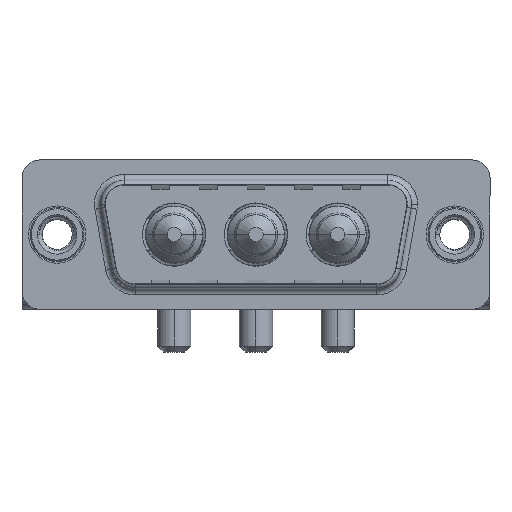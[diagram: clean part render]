
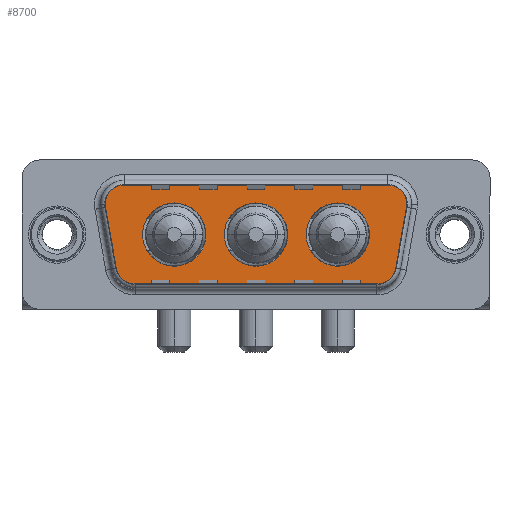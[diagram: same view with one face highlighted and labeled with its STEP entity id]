
A CAD part, top view. The second image highlights one B-rep face of the part: STEP entity #8700.
In plain terms, the highlighted planar face has unit normal (0, 0, 1).
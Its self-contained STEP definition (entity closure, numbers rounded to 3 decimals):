
#9 = CARTESIAN_POINT ( 'NONE',  ( 23.5, 0., 0. ) ) ;
#23 = CARTESIAN_POINT ( 'NONE',  ( 29.859, 2.553, 0. ) ) ;
#68 = CARTESIAN_POINT ( 'NONE',  ( 7.15, 0., 0. ) ) ;
#127 = CARTESIAN_POINT ( 'NONE',  ( 26.15, 0., 0. ) ) ;
#294 = DIRECTION ( 'NONE',  ( 0., 0., 1. ) ) ;
#381 = DIRECTION ( 'NONE',  ( 1., 0., 0. ) ) ;
#817 = EDGE_CURVE ( 'NONE', #10011, #8475, #13038, .T. ) ;
#833 = DIRECTION ( 'NONE',  ( 1., 0., 0. ) ) ;
#836 = EDGE_CURVE ( 'NONE', #10369, #5681, #14998, .T. ) ;
#904 = CIRCLE ( 'NONE', #12830, 2.65 ) ;
#1155 = AXIS2_PLACEMENT_3D ( 'NONE', #2225, #6966, #15307 ) ;
#1267 = CARTESIAN_POINT ( 'NONE',  ( 29.889, 2.9, 0. ) ) ;
#1299 = ORIENTED_EDGE ( 'NONE', *, *, #836, .T. ) ;
#1435 = CARTESIAN_POINT ( 'NONE',  ( 26.866, -4.9, 0. ) ) ;
#1461 = ORIENTED_EDGE ( 'NONE', *, *, #11948, .T. ) ;
#1512 = CIRCLE ( 'NONE', #6464, 2. ) ;
#1799 = EDGE_LOOP ( 'NONE', ( #3081, #1461, #11529, #5918, #14019, #12691, #6817, #14729, #1299 ) ) ;
#1834 = VERTEX_POINT ( 'NONE', #5460 ) ;
#1970 = EDGE_CURVE ( 'NONE', #3866, #10369, #1512, .T. ) ;
#2027 = VERTEX_POINT ( 'NONE', #13457 ) ;
#2169 = CARTESIAN_POINT ( 'NONE',  ( 5.411, 4.9, 0. ) ) ;
#2188 = AXIS2_PLACEMENT_3D ( 'NONE', #6352, #7614, #15015 ) ;
#2225 = CARTESIAN_POINT ( 'NONE',  ( 26.866, -2.9, 0. ) ) ;
#2233 = EDGE_CURVE ( 'NONE', #1834, #3443, #10955, .T. ) ;
#2374 = VECTOR ( 'NONE', #9341, 1000. ) ;
#2638 = CARTESIAN_POINT ( 'NONE',  ( 26.866, -2.9, 0. ) ) ;
#2776 = DIRECTION ( 'NONE',  ( 1., 0., 0. ) ) ;
#2869 = CARTESIAN_POINT ( 'NONE',  ( 19.3, 0., 0. ) ) ;
#3081 = ORIENTED_EDGE ( 'NONE', *, *, #5505, .T. ) ;
#3117 = ORIENTED_EDGE ( 'NONE', *, *, #9823, .F. ) ;
#3417 = DIRECTION ( 'NONE',  ( 0., 0., 1. ) ) ;
#3424 = CARTESIAN_POINT ( 'NONE',  ( 14., 0., 0. ) ) ;
#3443 = VERTEX_POINT ( 'NONE', #68 ) ;
#3513 = VERTEX_POINT ( 'NONE', #12124 ) ;
#3814 = FACE_BOUND ( 'NONE', #7966, .T. ) ;
#3866 = VERTEX_POINT ( 'NONE', #4338 ) ;
#3917 = CARTESIAN_POINT ( 'NONE',  ( 3.441, 2.553, 0. ) ) ;
#4032 = CARTESIAN_POINT ( 'NONE',  ( 5.411, 2.9, 0. ) ) ;
#4164 = VERTEX_POINT ( 'NONE', #4948 ) ;
#4166 = CIRCLE ( 'NONE', #2188, 2. ) ;
#4332 = CARTESIAN_POINT ( 'NONE',  ( 6.434, -4.9, 0. ) ) ;
#4338 = CARTESIAN_POINT ( 'NONE',  ( 4.464, -3.247, 0. ) ) ;
#4465 = CARTESIAN_POINT ( 'NONE',  ( 16.65, 0., 0. ) ) ;
#4595 = CARTESIAN_POINT ( 'NONE',  ( 6.434, -4.9, 0. ) ) ;
#4602 = CARTESIAN_POINT ( 'NONE',  ( 6.434, -2.9, 0. ) ) ;
#4746 = CARTESIAN_POINT ( 'NONE',  ( 16.65, 0., 0. ) ) ;
#4827 = CARTESIAN_POINT ( 'NONE',  ( 27.889, 4.9, 0. ) ) ;
#4946 = DIRECTION ( 'NONE',  ( 0.174, -0.985, 0. ) ) ;
#4948 = CARTESIAN_POINT ( 'NONE',  ( 20.85, 0., 0. ) ) ;
#4985 = EDGE_CURVE ( 'NONE', #13794, #3513, #14086, .T. ) ;
#5131 = CIRCLE ( 'NONE', #13845, 2.65 ) ;
#5460 = CARTESIAN_POINT ( 'NONE',  ( 12.45, 0., 0. ) ) ;
#5505 = EDGE_CURVE ( 'NONE', #5681, #9298, #15074, .T. ) ;
#5681 = VERTEX_POINT ( 'NONE', #1435 ) ;
#5796 = CARTESIAN_POINT ( 'NONE',  ( 27.889, 2.9, 0. ) ) ;
#5821 = DIRECTION ( 'NONE',  ( 1., 0., 0. ) ) ;
#5832 = AXIS2_PLACEMENT_3D ( 'NONE', #5796, #13989, #10556 ) ;
#5918 = ORIENTED_EDGE ( 'NONE', *, *, #12123, .T. ) ;
#5924 = DIRECTION ( 'NONE',  ( 0., 0., 1. ) ) ;
#5978 = AXIS2_PLACEMENT_3D ( 'NONE', #6756, #11443, #11521 ) ;
#6019 = EDGE_CURVE ( 'NONE', #3513, #2027, #15088, .T. ) ;
#6352 = CARTESIAN_POINT ( 'NONE',  ( 27.889, 2.9, 0. ) ) ;
#6464 = AXIS2_PLACEMENT_3D ( 'NONE', #4602, #5924, #9364 ) ;
#6468 = EDGE_CURVE ( 'NONE', #8916, #11478, #13773, .T. ) ;
#6756 = CARTESIAN_POINT ( 'NONE',  ( 9.8, 0., 0. ) ) ;
#6817 = ORIENTED_EDGE ( 'NONE', *, *, #7096, .T. ) ;
#6966 = DIRECTION ( 'NONE',  ( 0., 0., 1. ) ) ;
#7051 = AXIS2_PLACEMENT_3D ( 'NONE', #4746, #3417, #5821 ) ;
#7096 = EDGE_CURVE ( 'NONE', #2027, #3866, #8674, .T. ) ;
#7401 = DIRECTION ( 'NONE',  ( 0., 0., 1. ) ) ;
#7614 = DIRECTION ( 'NONE',  ( 0., 0., 1. ) ) ;
#7818 = CARTESIAN_POINT ( 'NONE',  ( 28.836, -3.247, 0. ) ) ;
#7966 = EDGE_LOOP ( 'NONE', ( #8834, #9786 ) ) ;
#8258 = LINE ( 'NONE', #14330, #8653 ) ;
#8325 = DIRECTION ( 'NONE',  ( 0., 0., 1. ) ) ;
#8475 = VERTEX_POINT ( 'NONE', #1267 ) ;
#8562 = FACE_OUTER_BOUND ( 'NONE', #1799, .T. ) ;
#8646 = DIRECTION ( 'NONE',  ( 1., 0., 0. ) ) ;
#8653 = VECTOR ( 'NONE', #14102, 1000. ) ;
#8674 = LINE ( 'NONE', #3917, #9735 ) ;
#8700 = ADVANCED_FACE ( 'NONE', ( #11136, #9753, #3814, #8562 ), #13305, .T. ) ;
#8834 = ORIENTED_EDGE ( 'NONE', *, *, #2233, .F. ) ;
#8868 = CIRCLE ( 'NONE', #15355, 2.65 ) ;
#8916 = VERTEX_POINT ( 'NONE', #3424 ) ;
#9030 = ORIENTED_EDGE ( 'NONE', *, *, #15248, .F. ) ;
#9217 = DIRECTION ( 'NONE',  ( 0., 0., 1. ) ) ;
#9298 = VERTEX_POINT ( 'NONE', #7818 ) ;
#9341 = DIRECTION ( 'NONE',  ( -1., 0., 0. ) ) ;
#9364 = DIRECTION ( 'NONE',  ( -1., 0., 0. ) ) ;
#9735 = VECTOR ( 'NONE', #4946, 1000. ) ;
#9753 = FACE_BOUND ( 'NONE', #13409, .T. ) ;
#9786 = ORIENTED_EDGE ( 'NONE', *, *, #12511, .F. ) ;
#9823 = EDGE_CURVE ( 'NONE', #11478, #8916, #904, .T. ) ;
#10011 = VERTEX_POINT ( 'NONE', #23 ) ;
#10038 = DIRECTION ( 'NONE',  ( 1., 0., 0. ) ) ;
#10240 = DIRECTION ( 'NONE',  ( 1., 0., 0. ) ) ;
#10369 = VERTEX_POINT ( 'NONE', #4595 ) ;
#10556 = DIRECTION ( 'NONE',  ( -1., 0., 0. ) ) ;
#10752 = EDGE_CURVE ( 'NONE', #14278, #4164, #5131, .T. ) ;
#10955 = CIRCLE ( 'NONE', #5978, 2.65 ) ;
#11136 = FACE_BOUND ( 'NONE', #13662, .T. ) ;
#11279 = DIRECTION ( 'NONE',  ( 0., 0., 1. ) ) ;
#11443 = DIRECTION ( 'NONE',  ( 0., 0., 1. ) ) ;
#11478 = VERTEX_POINT ( 'NONE', #2869 ) ;
#11521 = DIRECTION ( 'NONE',  ( 1., 0., 0. ) ) ;
#11529 = ORIENTED_EDGE ( 'NONE', *, *, #817, .T. ) ;
#11650 = AXIS2_PLACEMENT_3D ( 'NONE', #13597, #294, #13365 ) ;
#11948 = EDGE_CURVE ( 'NONE', #9298, #10011, #8258, .T. ) ;
#11972 = ORIENTED_EDGE ( 'NONE', *, *, #6468, .F. ) ;
#12123 = EDGE_CURVE ( 'NONE', #8475, #13794, #4166, .T. ) ;
#12124 = CARTESIAN_POINT ( 'NONE',  ( 5.411, 4.9, 0. ) ) ;
#12274 = AXIS2_PLACEMENT_3D ( 'NONE', #4032, #11279, #381 ) ;
#12511 = EDGE_CURVE ( 'NONE', #3443, #1834, #12647, .T. ) ;
#12647 = CIRCLE ( 'NONE', #11650, 2.65 ) ;
#12691 = ORIENTED_EDGE ( 'NONE', *, *, #6019, .T. ) ;
#12830 = AXIS2_PLACEMENT_3D ( 'NONE', #4465, #9217, #10240 ) ;
#12985 = AXIS2_PLACEMENT_3D ( 'NONE', #2638, #7401, #8646 ) ;
#13038 = CIRCLE ( 'NONE', #5832, 2. ) ;
#13305 = PLANE ( 'NONE',  #12985 ) ;
#13365 = DIRECTION ( 'NONE',  ( 1., 0., 0. ) ) ;
#13409 = EDGE_LOOP ( 'NONE', ( #13792, #9030 ) ) ;
#13457 = CARTESIAN_POINT ( 'NONE',  ( 3.441, 2.553, 0. ) ) ;
#13597 = CARTESIAN_POINT ( 'NONE',  ( 9.8, 0., 0. ) ) ;
#13662 = EDGE_LOOP ( 'NONE', ( #3117, #11972 ) ) ;
#13681 = CARTESIAN_POINT ( 'NONE',  ( 23.5, 0., 0. ) ) ;
#13773 = CIRCLE ( 'NONE', #7051, 2.65 ) ;
#13792 = ORIENTED_EDGE ( 'NONE', *, *, #10752, .F. ) ;
#13794 = VERTEX_POINT ( 'NONE', #4827 ) ;
#13845 = AXIS2_PLACEMENT_3D ( 'NONE', #13681, #14862, #10038 ) ;
#13989 = DIRECTION ( 'NONE',  ( 0., 0., 1. ) ) ;
#14019 = ORIENTED_EDGE ( 'NONE', *, *, #4985, .T. ) ;
#14044 = VECTOR ( 'NONE', #833, 1000. ) ;
#14086 = LINE ( 'NONE', #2169, #2374 ) ;
#14102 = DIRECTION ( 'NONE',  ( 0.174, 0.985, 0. ) ) ;
#14278 = VERTEX_POINT ( 'NONE', #127 ) ;
#14330 = CARTESIAN_POINT ( 'NONE',  ( 29.859, 2.553, 0. ) ) ;
#14729 = ORIENTED_EDGE ( 'NONE', *, *, #1970, .T. ) ;
#14862 = DIRECTION ( 'NONE',  ( 0., 0., 1. ) ) ;
#14998 = LINE ( 'NONE', #4332, #14044 ) ;
#15015 = DIRECTION ( 'NONE',  ( -1., 0., 0. ) ) ;
#15074 = CIRCLE ( 'NONE', #1155, 2. ) ;
#15088 = CIRCLE ( 'NONE', #12274, 2. ) ;
#15248 = EDGE_CURVE ( 'NONE', #4164, #14278, #8868, .T. ) ;
#15307 = DIRECTION ( 'NONE',  ( 1., 0., 0. ) ) ;
#15355 = AXIS2_PLACEMENT_3D ( 'NONE', #9, #8325, #2776 ) ;
